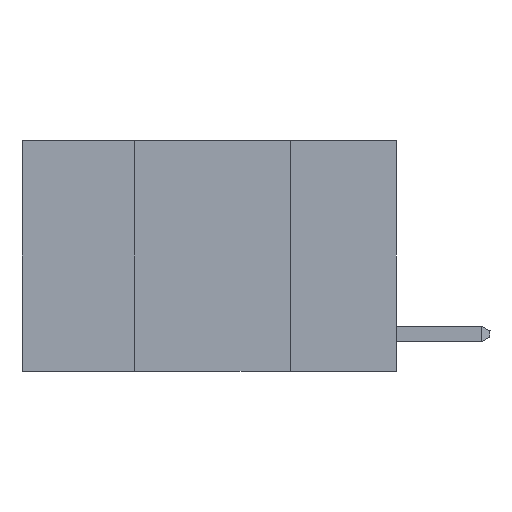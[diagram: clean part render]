
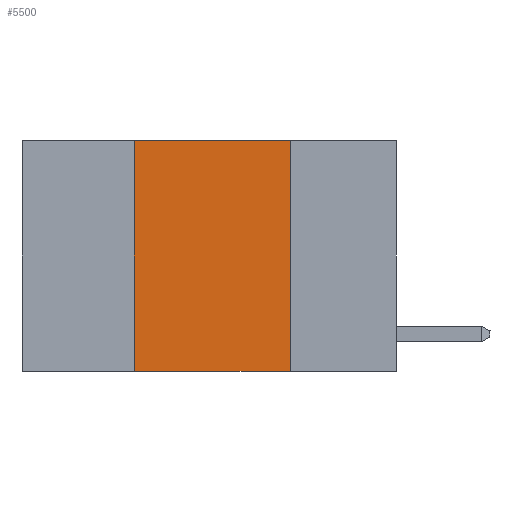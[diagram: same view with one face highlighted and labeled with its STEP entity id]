
A CAD part, left-side view. The second image highlights one B-rep face of the part: STEP entity #5500.
In plain terms, the highlighted planar face has unit normal (-1, 0, 0).
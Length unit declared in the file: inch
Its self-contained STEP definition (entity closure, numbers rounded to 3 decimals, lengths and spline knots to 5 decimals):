
#328 = VECTOR ( 'NONE', #9666, 39.37008 ) ;
#446 = CARTESIAN_POINT ( 'NONE',  ( 0., 0.42, 0. ) ) ;
#1235 = LINE ( 'NONE', #5553, #328 ) ;
#1510 = EDGE_LOOP ( 'NONE', ( #9201, #9159, #6231, #3727 ) ) ;
#1587 = VERTEX_POINT ( 'NONE', #3747 ) ;
#1896 = CARTESIAN_POINT ( 'NONE',  ( 0., 0.17, 0. ) ) ;
#2191 = DIRECTION ( 'NONE',  ( 0., 0., 1. ) ) ;
#2611 = DIRECTION ( 'NONE',  ( 0., 0., -1. ) ) ;
#2779 = AXIS2_PLACEMENT_3D ( 'NONE', #3299, #7517, #2611 ) ;
#3049 = LINE ( 'NONE', #5965, #5737 ) ;
#3299 = CARTESIAN_POINT ( 'NONE',  ( 0., 0.6, 0. ) ) ;
#3563 = EDGE_CURVE ( 'NONE', #8659, #1587, #4071, .T. ) ;
#3727 = ORIENTED_EDGE ( 'NONE', *, *, #8713, .T. ) ;
#3747 = CARTESIAN_POINT ( 'NONE',  ( 0., 0.42, 0. ) ) ;
#4060 = VECTOR ( 'NONE', #2191, 39.37008 ) ;
#4071 = LINE ( 'NONE', #446, #4060 ) ;
#4620 = CARTESIAN_POINT ( 'NONE',  ( 0., 0.6, 0. ) ) ;
#4919 = FACE_OUTER_BOUND ( 'NONE', #1510, .T. ) ;
#5156 = DIRECTION ( 'NONE',  ( 0., 0., -1. ) ) ;
#5479 = CARTESIAN_POINT ( 'NONE',  ( 0., 0.42, -0.37 ) ) ;
#5500 = ADVANCED_FACE ( 'NONE', ( #4919 ), #5873, .F. ) ;
#5553 = CARTESIAN_POINT ( 'NONE',  ( 0., 0.6, -0.37 ) ) ;
#5737 = VECTOR ( 'NONE', #5156, 39.37008 ) ;
#5873 = PLANE ( 'NONE',  #2779 ) ;
#5882 = LINE ( 'NONE', #4620, #7149 ) ;
#5965 = CARTESIAN_POINT ( 'NONE',  ( 0., 0.17, 0. ) ) ;
#6231 = ORIENTED_EDGE ( 'NONE', *, *, #3563, .F. ) ;
#6258 = CARTESIAN_POINT ( 'NONE',  ( 0., 0.17, -0.37 ) ) ;
#7132 = DIRECTION ( 'NONE',  ( 0., -1., 0. ) ) ;
#7149 = VECTOR ( 'NONE', #7132, 39.37008 ) ;
#7459 = EDGE_CURVE ( 'NONE', #1587, #7795, #5882, .T. ) ;
#7517 = DIRECTION ( 'NONE',  ( 1., 0., 0. ) ) ;
#7795 = VERTEX_POINT ( 'NONE', #1896 ) ;
#7803 = VERTEX_POINT ( 'NONE', #6258 ) ;
#8233 = EDGE_CURVE ( 'NONE', #7795, #7803, #3049, .T. ) ;
#8659 = VERTEX_POINT ( 'NONE', #5479 ) ;
#8713 = EDGE_CURVE ( 'NONE', #8659, #7803, #1235, .T. ) ;
#9159 = ORIENTED_EDGE ( 'NONE', *, *, #7459, .F. ) ;
#9201 = ORIENTED_EDGE ( 'NONE', *, *, #8233, .F. ) ;
#9666 = DIRECTION ( 'NONE',  ( 0., -1., 0. ) ) ;
